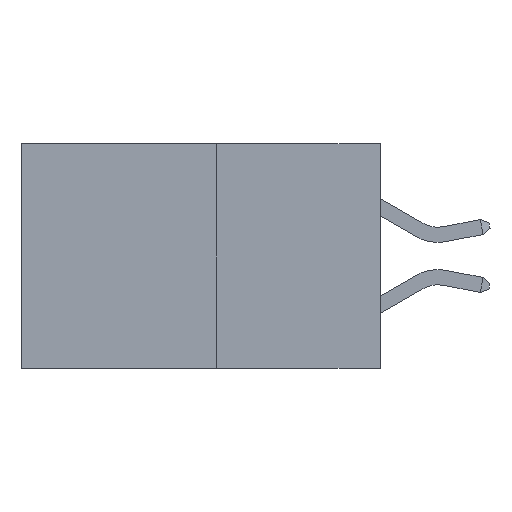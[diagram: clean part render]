
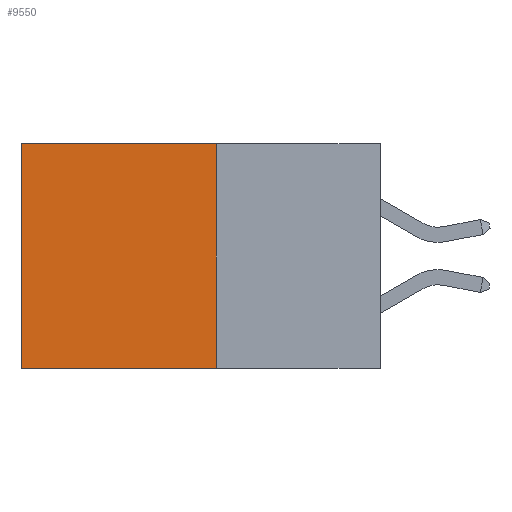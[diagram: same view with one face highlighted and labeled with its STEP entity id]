
A CAD part, left-side view. The second image highlights one B-rep face of the part: STEP entity #9550.
In plain terms, the highlighted planar face has unit normal (-1, 0, 0).
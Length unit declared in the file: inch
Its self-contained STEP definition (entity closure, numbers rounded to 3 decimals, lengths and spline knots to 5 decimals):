
#223 = ORIENTED_EDGE ( 'NONE', *, *, #25293, .T. ) ;
#412 = VECTOR ( 'NONE', #9588, 39.37008 ) ;
#840 = DIRECTION ( 'NONE',  ( 0., 0., -1. ) ) ;
#1668 = EDGE_LOOP ( 'NONE', ( #223, #10624, #14795, #3808 ) ) ;
#2426 = VERTEX_POINT ( 'NONE', #16161 ) ;
#3213 = VECTOR ( 'NONE', #21937, 39.37008 ) ;
#3808 = ORIENTED_EDGE ( 'NONE', *, *, #15452, .T. ) ;
#4404 = VECTOR ( 'NONE', #19614, 39.37008 ) ;
#4495 = LINE ( 'NONE', #11728, #3213 ) ;
#4637 = AXIS2_PLACEMENT_3D ( 'NONE', #18105, #24217, #11956 ) ;
#5188 = CARTESIAN_POINT ( 'NONE',  ( 0.277, 0.27, 0. ) ) ;
#5805 = VERTEX_POINT ( 'NONE', #13861 ) ;
#5971 = LINE ( 'NONE', #23873, #412 ) ;
#6854 = LINE ( 'NONE', #25486, #17172 ) ;
#8564 = CARTESIAN_POINT ( 'NONE',  ( 0.277, 0.59, 0. ) ) ;
#9550 = ADVANCED_FACE ( 'NONE', ( #20366 ), #22158, .F. ) ;
#9588 = DIRECTION ( 'NONE',  ( 0., 1., 0. ) ) ;
#9593 = CARTESIAN_POINT ( 'NONE',  ( 0.277, 0.27, -0.37 ) ) ;
#10624 = ORIENTED_EDGE ( 'NONE', *, *, #16996, .F. ) ;
#11728 = CARTESIAN_POINT ( 'NONE',  ( 0.277, 0.59, -0.37 ) ) ;
#11956 = DIRECTION ( 'NONE',  ( 0., 0., -1. ) ) ;
#12430 = VERTEX_POINT ( 'NONE', #9593 ) ;
#12875 = EDGE_CURVE ( 'NONE', #5805, #12430, #6854, .T. ) ;
#13359 = VERTEX_POINT ( 'NONE', #8564 ) ;
#13861 = CARTESIAN_POINT ( 'NONE',  ( 0.277, 0.27, 0. ) ) ;
#14795 = ORIENTED_EDGE ( 'NONE', *, *, #12875, .F. ) ;
#15452 = EDGE_CURVE ( 'NONE', #5805, #13359, #20839, .T. ) ;
#16161 = CARTESIAN_POINT ( 'NONE',  ( 0.277, 0.59, -0.37 ) ) ;
#16996 = EDGE_CURVE ( 'NONE', #12430, #2426, #5971, .T. ) ;
#17172 = VECTOR ( 'NONE', #840, 39.37008 ) ;
#18105 = CARTESIAN_POINT ( 'NONE',  ( 0.277, 0.27, -0.37 ) ) ;
#19614 = DIRECTION ( 'NONE',  ( 0., 1., 0. ) ) ;
#20366 = FACE_OUTER_BOUND ( 'NONE', #1668, .T. ) ;
#20839 = LINE ( 'NONE', #5188, #4404 ) ;
#21937 = DIRECTION ( 'NONE',  ( 0., 0., -1. ) ) ;
#22158 = PLANE ( 'NONE',  #4637 ) ;
#23873 = CARTESIAN_POINT ( 'NONE',  ( 0.277, 0.27, -0.37 ) ) ;
#24217 = DIRECTION ( 'NONE',  ( 1., 0., 0. ) ) ;
#25293 = EDGE_CURVE ( 'NONE', #13359, #2426, #4495, .T. ) ;
#25486 = CARTESIAN_POINT ( 'NONE',  ( 0.277, 0.27, -0.37 ) ) ;
